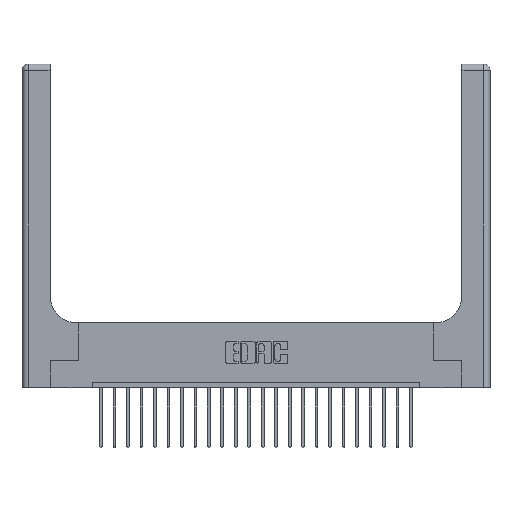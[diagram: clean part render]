
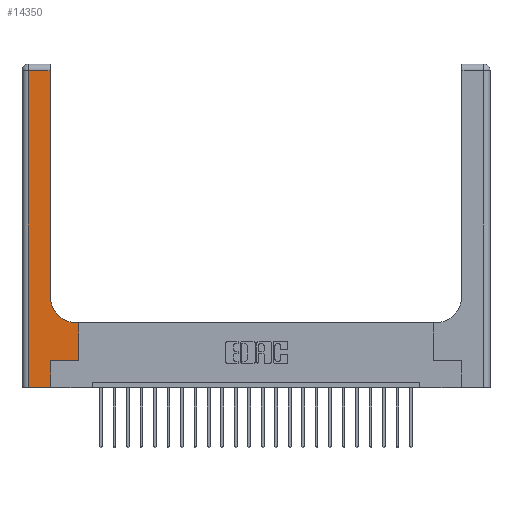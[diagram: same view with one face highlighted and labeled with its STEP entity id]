
A CAD part, top view. The second image highlights one B-rep face of the part: STEP entity #14350.
In plain terms, the highlighted planar face has unit normal (0, 0, 1).
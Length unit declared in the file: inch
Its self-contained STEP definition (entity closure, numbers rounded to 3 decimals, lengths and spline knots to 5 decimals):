
#475 = DIRECTION ( 'NONE',  ( -1., 0., 0. ) ) ;
#2058 = LINE ( 'NONE', #9148, #20200 ) ;
#2224 = ORIENTED_EDGE ( 'NONE', *, *, #17840, .T. ) ;
#2273 = ORIENTED_EDGE ( 'NONE', *, *, #17244, .T. ) ;
#2595 = VERTEX_POINT ( 'NONE', #10758 ) ;
#2847 = EDGE_CURVE ( 'NONE', #16100, #17999, #3178, .T. ) ;
#3178 = LINE ( 'NONE', #11665, #7140 ) ;
#3277 = ORIENTED_EDGE ( 'NONE', *, *, #2847, .T. ) ;
#3744 = CARTESIAN_POINT ( 'NONE',  ( 0.265, 0.25, 0.37 ) ) ;
#3779 = DIRECTION ( 'NONE',  ( 1., 0., 0. ) ) ;
#3916 = EDGE_CURVE ( 'NONE', #2595, #10423, #21551, .T. ) ;
#5002 = DIRECTION ( 'NONE',  ( -1., 0., 0. ) ) ;
#5371 = CARTESIAN_POINT ( 'NONE',  ( 0., 2.94, 0.37 ) ) ;
#6165 = VECTOR ( 'NONE', #14296, 39.37008 ) ;
#6626 = LINE ( 'NONE', #21047, #8672 ) ;
#6652 = EDGE_CURVE ( 'NONE', #10208, #16100, #14177, .T. ) ;
#7140 = VECTOR ( 'NONE', #8071, 39.37008 ) ;
#7208 = EDGE_CURVE ( 'NONE', #11182, #13205, #20518, .T. ) ;
#7388 = CARTESIAN_POINT ( 'NONE',  ( 0., 0., 0.37 ) ) ;
#7559 = VECTOR ( 'NONE', #3779, 39.37008 ) ;
#7770 = DIRECTION ( 'NONE',  ( 0., 0., -1. ) ) ;
#8071 = DIRECTION ( 'NONE',  ( 0., -1., 0. ) ) ;
#8672 = VECTOR ( 'NONE', #5002, 39.37008 ) ;
#8725 = CARTESIAN_POINT ( 'NONE',  ( 0., 3., 0.37 ) ) ;
#8879 = DIRECTION ( 'NONE',  ( 0., 1., 0. ) ) ;
#9148 = CARTESIAN_POINT ( 'NONE',  ( 0.265, 0.25, 0.37 ) ) ;
#10208 = VERTEX_POINT ( 'NONE', #14921 ) ;
#10423 = VERTEX_POINT ( 'NONE', #3744 ) ;
#10471 = PLANE ( 'NONE',  #17476 ) ;
#10758 = CARTESIAN_POINT ( 'NONE',  ( 0.265, 0., 0.37 ) ) ;
#10909 = CARTESIAN_POINT ( 'NONE',  ( 0.51, 0.6, 0.37 ) ) ;
#11182 = VERTEX_POINT ( 'NONE', #11846 ) ;
#11665 = CARTESIAN_POINT ( 'NONE',  ( 0.06, 3., 0.37 ) ) ;
#11732 = ORIENTED_EDGE ( 'NONE', *, *, #7208, .T. ) ;
#11846 = CARTESIAN_POINT ( 'NONE',  ( 0.528, 0.25, 0.37 ) ) ;
#12128 = CARTESIAN_POINT ( 'NONE',  ( 0.26, 3., 0.37 ) ) ;
#12254 = AXIS2_PLACEMENT_3D ( 'NONE', #13143, #12919, #16872 ) ;
#12517 = ORIENTED_EDGE ( 'NONE', *, *, #3916, .T. ) ;
#12919 = DIRECTION ( 'NONE',  ( 0., 0., -1. ) ) ;
#13143 = CARTESIAN_POINT ( 'NONE',  ( 0.51, 0.85, 0.37 ) ) ;
#13205 = VERTEX_POINT ( 'NONE', #15380 ) ;
#13497 = EDGE_CURVE ( 'NONE', #20704, #21285, #21557, .T. ) ;
#13555 = ORIENTED_EDGE ( 'NONE', *, *, #13497, .T. ) ;
#14177 = LINE ( 'NONE', #5371, #6165 ) ;
#14296 = DIRECTION ( 'NONE',  ( -1., 0., 0. ) ) ;
#14332 = VECTOR ( 'NONE', #18772, 39.37008 ) ;
#14350 = ADVANCED_FACE ( 'NONE', ( #18004 ), #10471, .F. ) ;
#14921 = CARTESIAN_POINT ( 'NONE',  ( 0.26, 2.94, 0.37 ) ) ;
#15082 = ORIENTED_EDGE ( 'NONE', *, *, #6652, .T. ) ;
#15303 = EDGE_CURVE ( 'NONE', #21285, #10208, #20975, .T. ) ;
#15380 = CARTESIAN_POINT ( 'NONE',  ( 0.528, 0.6, 0.37 ) ) ;
#15468 = VECTOR ( 'NONE', #19800, 39.37008 ) ;
#15892 = CARTESIAN_POINT ( 'NONE',  ( 0.06, 2.94, 0.37 ) ) ;
#16100 = VERTEX_POINT ( 'NONE', #15892 ) ;
#16327 = DIRECTION ( 'NONE',  ( 1., 0., 0. ) ) ;
#16586 = ORIENTED_EDGE ( 'NONE', *, *, #15303, .T. ) ;
#16738 = VECTOR ( 'NONE', #8879, 39.37008 ) ;
#16832 = ORIENTED_EDGE ( 'NONE', *, *, #21081, .T. ) ;
#16872 = DIRECTION ( 'NONE',  ( 1., 0., 0. ) ) ;
#17244 = EDGE_CURVE ( 'NONE', #13205, #20704, #6626, .T. ) ;
#17476 = AXIS2_PLACEMENT_3D ( 'NONE', #8725, #7770, #475 ) ;
#17838 = LINE ( 'NONE', #7388, #7559 ) ;
#17840 = EDGE_CURVE ( 'NONE', #10423, #11182, #2058, .T. ) ;
#17999 = VERTEX_POINT ( 'NONE', #18783 ) ;
#18004 = FACE_OUTER_BOUND ( 'NONE', #22877, .T. ) ;
#18772 = DIRECTION ( 'NONE',  ( 0., 1., 0. ) ) ;
#18783 = CARTESIAN_POINT ( 'NONE',  ( 0.06, 0., 0.37 ) ) ;
#18891 = CARTESIAN_POINT ( 'NONE',  ( 0.26, 0.85, 0.37 ) ) ;
#19683 = CARTESIAN_POINT ( 'NONE',  ( 0.265, 0., 0.37 ) ) ;
#19800 = DIRECTION ( 'NONE',  ( 0., 1., 0. ) ) ;
#20200 = VECTOR ( 'NONE', #16327, 39.37008 ) ;
#20403 = CARTESIAN_POINT ( 'NONE',  ( 0.528, 0.25, 0.37 ) ) ;
#20518 = LINE ( 'NONE', #20403, #14332 ) ;
#20704 = VERTEX_POINT ( 'NONE', #10909 ) ;
#20975 = LINE ( 'NONE', #12128, #16738 ) ;
#21047 = CARTESIAN_POINT ( 'NONE',  ( 0.26, 0.6, 0.37 ) ) ;
#21081 = EDGE_CURVE ( 'NONE', #17999, #2595, #17838, .T. ) ;
#21285 = VERTEX_POINT ( 'NONE', #18891 ) ;
#21551 = LINE ( 'NONE', #19683, #15468 ) ;
#21557 = CIRCLE ( 'NONE', #12254, 0.25 ) ;
#22877 = EDGE_LOOP ( 'NONE', ( #16586, #15082, #3277, #16832, #12517, #2224, #11732, #2273, #13555 ) ) ;
